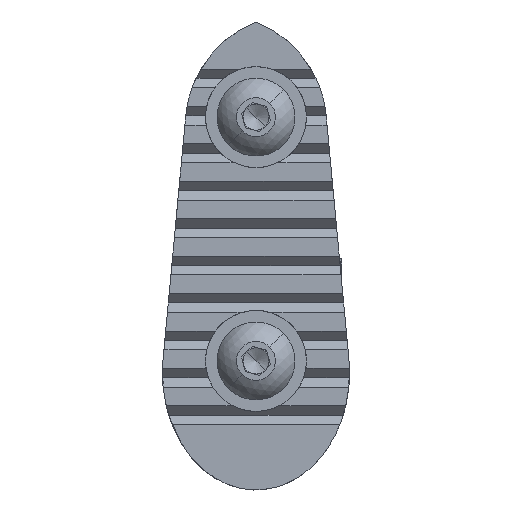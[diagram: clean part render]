
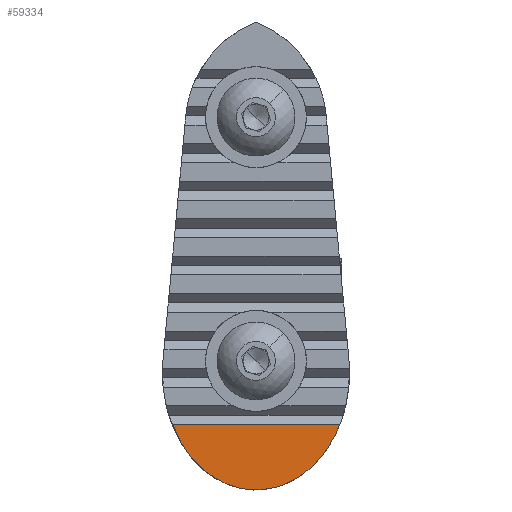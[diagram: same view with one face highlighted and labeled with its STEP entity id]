
A CAD part, top view. The second image highlights one B-rep face of the part: STEP entity #59334.
In plain terms, the highlighted planar face has unit normal (0, 0, 1).
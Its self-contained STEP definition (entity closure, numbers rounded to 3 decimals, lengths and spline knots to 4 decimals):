
#323 = EDGE_CURVE ( 'NONE', #2865, #29848, #64206, .T. ) ;
#495 = DIRECTION ( 'NONE',  ( 1., 0., 0. ) ) ;
#2865 = VERTEX_POINT ( 'NONE', #15344 ) ;
#6674 = LINE ( 'NONE', #31557, #47670 ) ;
#7061 = ORIENTED_EDGE ( 'NONE', *, *, #52722, .T. ) ;
#15344 = CARTESIAN_POINT ( 'NONE',  ( 0.7063, 0.9351, 0.7283 ) ) ;
#17973 = CARTESIAN_POINT ( 'NONE',  ( -0.7063, 0.9351, 0.7283 ) ) ;
#18818 = AXIS2_PLACEMENT_3D ( 'NONE', #63784, #48757, #22717 ) ;
#22717 = DIRECTION ( 'NONE',  ( 1., 0., 0. ) ) ;
#28751 = PLANE ( 'NONE',  #18818 ) ;
#29043 = CARTESIAN_POINT ( 'NONE',  ( 0.7063, 0.9351, 0.7283 ) ) ;
#29781 = EDGE_LOOP ( 'NONE', ( #7061, #66683 ) ) ;
#29848 = VERTEX_POINT ( 'NONE', #17973 ) ;
#31557 = CARTESIAN_POINT ( 'NONE',  ( -0.7874, 0.9351, 0.7283 ) ) ;
#33981 = CARTESIAN_POINT ( 'NONE',  ( -0.7063, 0.9351, 0.7283 ) ) ;
#39567 = CARTESIAN_POINT ( 'NONE',  ( -0.3749, 1.7757, 0.7283 ) ) ;
#44634 = FACE_OUTER_BOUND ( 'NONE', #29781, .T. ) ;
#47670 = VECTOR ( 'NONE', #495, 39.3701 ) ;
#48757 = DIRECTION ( 'NONE',  ( 0., 0., 1. ) ) ;
#52722 = EDGE_CURVE ( 'NONE', #29848, #2865, #6674, .T. ) ;
#55320 = CARTESIAN_POINT ( 'NONE',  ( 0.3749, 1.7757, 0.7283 ) ) ;
#59334 = ADVANCED_FACE ( 'NONE', ( #44634 ), #28751, .T. ) ;
#63784 = CARTESIAN_POINT ( 'NONE',  ( 0., 0.5, 0.7283 ) ) ;
#64206 =( BOUNDED_CURVE ( )  B_SPLINE_CURVE ( 3, ( #29043, #55320, #39567, #33981 ),
 .UNSPECIFIED., .F., .T. ) 
 B_SPLINE_CURVE_WITH_KNOTS ( ( 4, 4 ),
 ( 2.0287, 4.2545 ),
 .UNSPECIFIED. ) 
 CURVE ( )  GEOMETRIC_REPRESENTATION_ITEM ( )  RATIONAL_B_SPLINE_CURVE ( ( 1., 0.628, 0.628, 1. ) ) 
 REPRESENTATION_ITEM ( '' )  );
#66683 = ORIENTED_EDGE ( 'NONE', *, *, #323, .T. ) ;
